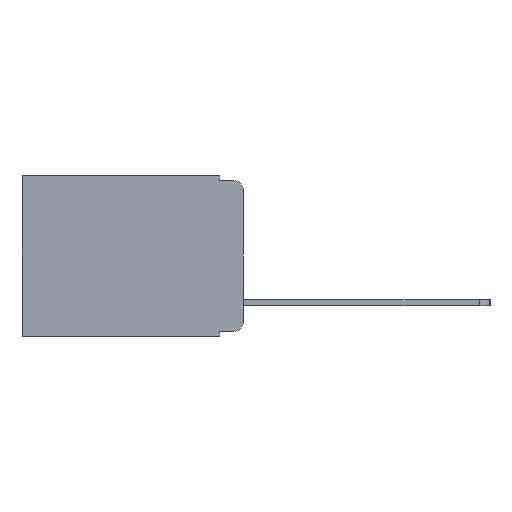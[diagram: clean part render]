
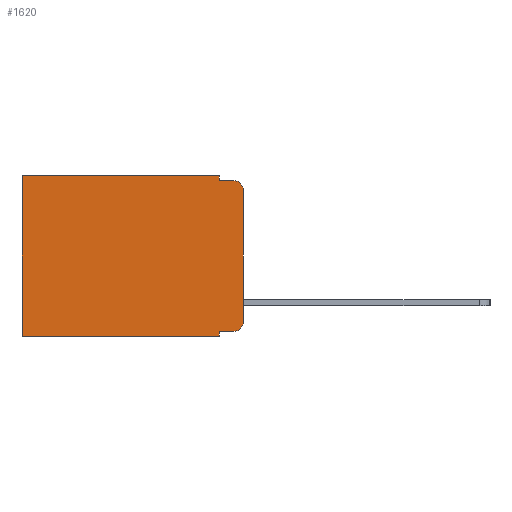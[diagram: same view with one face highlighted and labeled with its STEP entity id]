
A CAD part, left-side view. The second image highlights one B-rep face of the part: STEP entity #1620.
In plain terms, the highlighted planar face has unit normal (-1, 0, 0).
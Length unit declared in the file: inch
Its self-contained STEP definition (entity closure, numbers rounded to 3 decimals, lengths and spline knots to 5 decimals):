
#106 = LINE ( 'NONE', #10028, #4456 ) ;
#147 = FACE_OUTER_BOUND ( 'NONE', #7528, .T. ) ;
#339 = LINE ( 'NONE', #1900, #9157 ) ;
#421 = CARTESIAN_POINT ( 'NONE',  ( 0.298, 0., -0.343 ) ) ;
#520 = DIRECTION ( 'NONE',  ( 0., 0., -1. ) ) ;
#616 = EDGE_CURVE ( 'NONE', #1447, #1112, #339, .T. ) ;
#822 = DIRECTION ( 'NONE',  ( 0., -1., 0. ) ) ;
#886 = VERTEX_POINT ( 'NONE', #10212 ) ;
#1112 = VERTEX_POINT ( 'NONE', #2271 ) ;
#1225 = DIRECTION ( 'NONE',  ( 0., 0., -1. ) ) ;
#1447 = VERTEX_POINT ( 'NONE', #8304 ) ;
#1620 = ADVANCED_FACE ( 'NONE', ( #147 ), #8571, .F. ) ;
#1635 = VERTEX_POINT ( 'NONE', #5511 ) ;
#1636 = EDGE_CURVE ( 'NONE', #1635, #3301, #4237, .T. ) ;
#1900 = CARTESIAN_POINT ( 'NONE',  ( 0.298, 0., 0. ) ) ;
#2205 = EDGE_CURVE ( 'NONE', #3301, #8105, #7392, .T. ) ;
#2257 = ORIENTED_EDGE ( 'NONE', *, *, #5684, .T. ) ;
#2271 = CARTESIAN_POINT ( 'NONE',  ( 0.298, 0., -0.313 ) ) ;
#2708 = EDGE_CURVE ( 'NONE', #1635, #886, #9081, .T. ) ;
#2719 = ORIENTED_EDGE ( 'NONE', *, *, #5235, .F. ) ;
#2834 = VECTOR ( 'NONE', #520, 39.37008 ) ;
#2943 = CIRCLE ( 'NONE', #6216, 0.02 ) ;
#2981 = CARTESIAN_POINT ( 'NONE',  ( 0.298, 0.473, 0. ) ) ;
#3235 = VECTOR ( 'NONE', #10439, 39.37008 ) ;
#3301 = VERTEX_POINT ( 'NONE', #3990 ) ;
#3399 = EDGE_CURVE ( 'NONE', #4143, #1112, #2943, .T. ) ;
#3505 = LINE ( 'NONE', #10953, #9467 ) ;
#3887 = ORIENTED_EDGE ( 'NONE', *, *, #10301, .F. ) ;
#3990 = CARTESIAN_POINT ( 'NONE',  ( 0.298, 0.473, 0. ) ) ;
#4005 = VERTEX_POINT ( 'NONE', #6346 ) ;
#4143 = VERTEX_POINT ( 'NONE', #5686 ) ;
#4237 = LINE ( 'NONE', #8423, #10658 ) ;
#4360 = DIRECTION ( 'NONE',  ( 0., 0., -1. ) ) ;
#4456 = VECTOR ( 'NONE', #8360, 39.37008 ) ;
#4608 = CARTESIAN_POINT ( 'NONE',  ( 0.298, 0.02, -0.03 ) ) ;
#4884 = CARTESIAN_POINT ( 'NONE',  ( 0.298, 0.473, -0.343 ) ) ;
#5235 = EDGE_CURVE ( 'NONE', #886, #4005, #5260, .T. ) ;
#5260 = LINE ( 'NONE', #5410, #3235 ) ;
#5264 = DIRECTION ( 'NONE',  ( 0., 1., 0. ) ) ;
#5410 = CARTESIAN_POINT ( 'NONE',  ( 0.298, 0.051, -0.01 ) ) ;
#5423 = DIRECTION ( 'NONE',  ( 0., 0., -1. ) ) ;
#5511 = CARTESIAN_POINT ( 'NONE',  ( 0.298, 0.051, 0. ) ) ;
#5684 = EDGE_CURVE ( 'NONE', #9473, #4143, #3505, .T. ) ;
#5686 = CARTESIAN_POINT ( 'NONE',  ( 0.298, 0.02, -0.333 ) ) ;
#5862 = AXIS2_PLACEMENT_3D ( 'NONE', #4608, #10460, #5423 ) ;
#5912 = CARTESIAN_POINT ( 'NONE',  ( 0.298, 0.051, -0.333 ) ) ;
#5972 = DIRECTION ( 'NONE',  ( 0., 0., -1. ) ) ;
#5990 = CARTESIAN_POINT ( 'NONE',  ( 0.298, 0.051, 0. ) ) ;
#6196 = EDGE_CURVE ( 'NONE', #9473, #6269, #106, .T. ) ;
#6216 = AXIS2_PLACEMENT_3D ( 'NONE', #9299, #9264, #9227 ) ;
#6269 = VERTEX_POINT ( 'NONE', #7579 ) ;
#6343 = CIRCLE ( 'NONE', #5862, 0.02 ) ;
#6346 = CARTESIAN_POINT ( 'NONE',  ( 0.298, 0.02, -0.01 ) ) ;
#6431 = DIRECTION ( 'NONE',  ( 0., 1., 0. ) ) ;
#6650 = ORIENTED_EDGE ( 'NONE', *, *, #616, .F. ) ;
#6687 = ORIENTED_EDGE ( 'NONE', *, *, #6196, .F. ) ;
#6839 = VECTOR ( 'NONE', #5972, 39.37008 ) ;
#7340 = ORIENTED_EDGE ( 'NONE', *, *, #1636, .T. ) ;
#7392 = LINE ( 'NONE', #2981, #2834 ) ;
#7501 = AXIS2_PLACEMENT_3D ( 'NONE', #10121, #8578, #1225 ) ;
#7528 = EDGE_LOOP ( 'NONE', ( #6650, #10012, #2719, #9787, #7340, #8681, #3887, #6687, #2257, #8366 ) ) ;
#7579 = CARTESIAN_POINT ( 'NONE',  ( 0.298, 0.051, -0.343 ) ) ;
#8105 = VERTEX_POINT ( 'NONE', #4884 ) ;
#8304 = CARTESIAN_POINT ( 'NONE',  ( 0.298, 0., -0.03 ) ) ;
#8360 = DIRECTION ( 'NONE',  ( 0., 0., -1. ) ) ;
#8366 = ORIENTED_EDGE ( 'NONE', *, *, #3399, .T. ) ;
#8423 = CARTESIAN_POINT ( 'NONE',  ( 0.298, 0., 0. ) ) ;
#8571 = PLANE ( 'NONE',  #7501 ) ;
#8578 = DIRECTION ( 'NONE',  ( 1., 0., 0. ) ) ;
#8681 = ORIENTED_EDGE ( 'NONE', *, *, #2205, .T. ) ;
#8797 = VECTOR ( 'NONE', #6431, 39.37008 ) ;
#9081 = LINE ( 'NONE', #5990, #6839 ) ;
#9157 = VECTOR ( 'NONE', #4360, 39.37008 ) ;
#9227 = DIRECTION ( 'NONE',  ( 0., 0., -1. ) ) ;
#9264 = DIRECTION ( 'NONE',  ( -1., 0., 0. ) ) ;
#9299 = CARTESIAN_POINT ( 'NONE',  ( 0.298, 0.02, -0.313 ) ) ;
#9467 = VECTOR ( 'NONE', #822, 39.37008 ) ;
#9473 = VERTEX_POINT ( 'NONE', #5912 ) ;
#9747 = EDGE_CURVE ( 'NONE', #1447, #4005, #6343, .T. ) ;
#9787 = ORIENTED_EDGE ( 'NONE', *, *, #2708, .F. ) ;
#10012 = ORIENTED_EDGE ( 'NONE', *, *, #9747, .T. ) ;
#10028 = CARTESIAN_POINT ( 'NONE',  ( 0.298, 0.051, 0. ) ) ;
#10121 = CARTESIAN_POINT ( 'NONE',  ( 0.298, 0., 0. ) ) ;
#10212 = CARTESIAN_POINT ( 'NONE',  ( 0.298, 0.051, -0.01 ) ) ;
#10301 = EDGE_CURVE ( 'NONE', #6269, #8105, #10970, .T. ) ;
#10439 = DIRECTION ( 'NONE',  ( 0., -1., 0. ) ) ;
#10460 = DIRECTION ( 'NONE',  ( -1., 0., 0. ) ) ;
#10658 = VECTOR ( 'NONE', #5264, 39.37008 ) ;
#10953 = CARTESIAN_POINT ( 'NONE',  ( 0.298, 0.051, -0.333 ) ) ;
#10970 = LINE ( 'NONE', #421, #8797 ) ;
